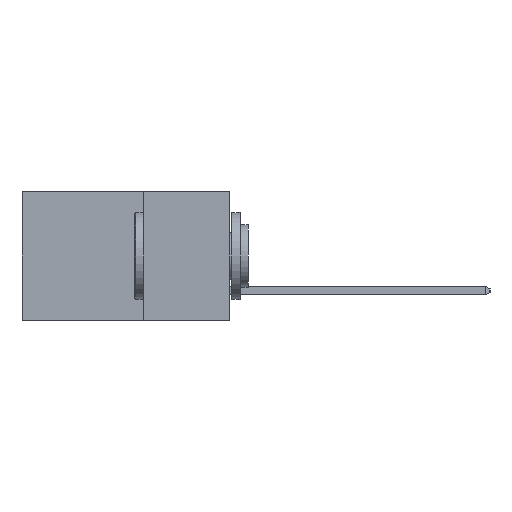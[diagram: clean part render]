
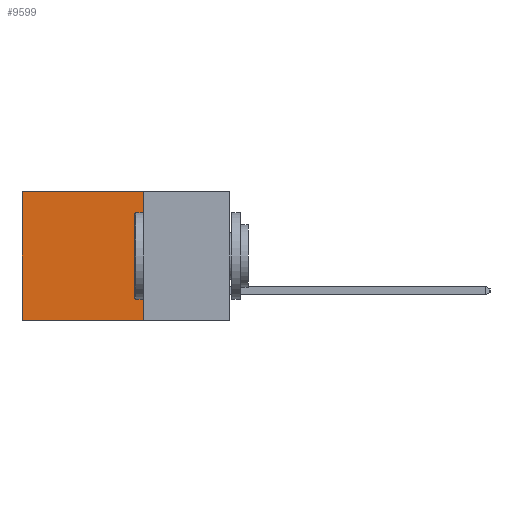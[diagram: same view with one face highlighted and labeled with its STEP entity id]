
A CAD part, left-side view. The second image highlights one B-rep face of the part: STEP entity #9599.
In plain terms, the highlighted planar face has unit normal (-1, 0, 0).
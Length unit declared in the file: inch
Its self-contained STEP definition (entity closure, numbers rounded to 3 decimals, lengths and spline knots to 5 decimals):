
#324 = LINE ( 'NONE', #4389, #10872 ) ;
#799 = DIRECTION ( 'NONE',  ( 1., 0., 0. ) ) ;
#1049 = AXIS2_PLACEMENT_3D ( 'NONE', #9392, #799, #10851 ) ;
#2038 = CARTESIAN_POINT ( 'NONE',  ( 0.298, 0.25, 0. ) ) ;
#2744 = DIRECTION ( 'NONE',  ( 0., 0., -1. ) ) ;
#3430 = EDGE_CURVE ( 'NONE', #11093, #16858, #14253, .T. ) ;
#4257 = EDGE_CURVE ( 'NONE', #16106, #15885, #18403, .T. ) ;
#4389 = CARTESIAN_POINT ( 'NONE',  ( 0.298, 0.25, 0. ) ) ;
#4490 = CARTESIAN_POINT ( 'NONE',  ( 0.298, 0.25, -0.37 ) ) ;
#5794 = EDGE_CURVE ( 'NONE', #15885, #16858, #17908, .T. ) ;
#5832 = DIRECTION ( 'NONE',  ( 0., 1., 0. ) ) ;
#6027 = CARTESIAN_POINT ( 'NONE',  ( 0.298, 0.6, 0. ) ) ;
#6064 = CARTESIAN_POINT ( 'NONE',  ( 0.298, 0.6, -0.37 ) ) ;
#6275 = VECTOR ( 'NONE', #2744, 39.37008 ) ;
#6688 = DIRECTION ( 'NONE',  ( 0., 0., -1. ) ) ;
#7337 = CARTESIAN_POINT ( 'NONE',  ( 0.298, 0.25, 0. ) ) ;
#7650 = ORIENTED_EDGE ( 'NONE', *, *, #5794, .F. ) ;
#8361 = DIRECTION ( 'NONE',  ( 0., 1., 0. ) ) ;
#9392 = CARTESIAN_POINT ( 'NONE',  ( 0.298, 0.25, 0. ) ) ;
#9599 = ADVANCED_FACE ( 'NONE', ( #12409 ), #12186, .F. ) ;
#9900 = EDGE_CURVE ( 'NONE', #16106, #11093, #324, .T. ) ;
#10096 = CARTESIAN_POINT ( 'NONE',  ( 0.298, 0.25, -0.37 ) ) ;
#10851 = DIRECTION ( 'NONE',  ( 0., 0., -1. ) ) ;
#10872 = VECTOR ( 'NONE', #5832, 39.37008 ) ;
#10953 = VECTOR ( 'NONE', #6688, 39.37008 ) ;
#11093 = VERTEX_POINT ( 'NONE', #11892 ) ;
#11892 = CARTESIAN_POINT ( 'NONE',  ( 0.298, 0.6, 0. ) ) ;
#12186 = PLANE ( 'NONE',  #1049 ) ;
#12409 = FACE_OUTER_BOUND ( 'NONE', #17102, .T. ) ;
#13485 = ORIENTED_EDGE ( 'NONE', *, *, #3430, .T. ) ;
#14167 = VECTOR ( 'NONE', #8361, 39.37008 ) ;
#14253 = LINE ( 'NONE', #6027, #6275 ) ;
#14633 = ORIENTED_EDGE ( 'NONE', *, *, #4257, .F. ) ;
#15885 = VERTEX_POINT ( 'NONE', #4490 ) ;
#16106 = VERTEX_POINT ( 'NONE', #2038 ) ;
#16858 = VERTEX_POINT ( 'NONE', #6064 ) ;
#17081 = ORIENTED_EDGE ( 'NONE', *, *, #9900, .T. ) ;
#17102 = EDGE_LOOP ( 'NONE', ( #13485, #7650, #14633, #17081 ) ) ;
#17908 = LINE ( 'NONE', #10096, #14167 ) ;
#18403 = LINE ( 'NONE', #7337, #10953 ) ;
